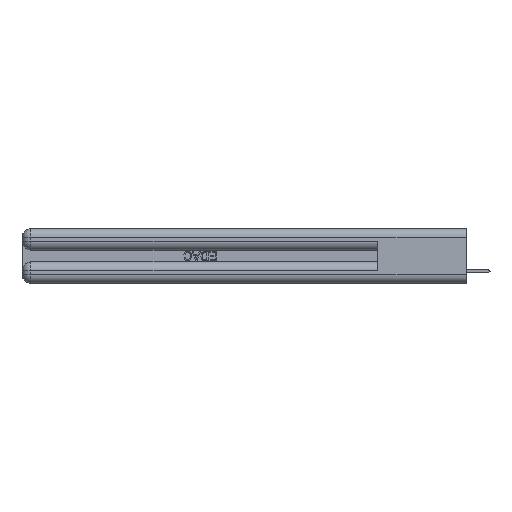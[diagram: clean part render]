
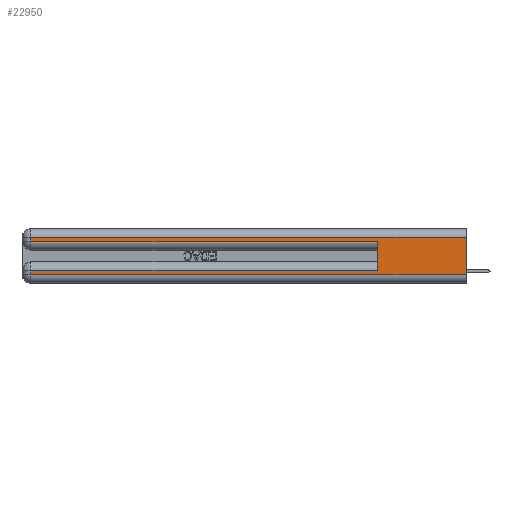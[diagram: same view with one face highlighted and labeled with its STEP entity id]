
A CAD part, left-side view. The second image highlights one B-rep face of the part: STEP entity #22950.
In plain terms, the highlighted planar face has unit normal (-1, 0, 0).
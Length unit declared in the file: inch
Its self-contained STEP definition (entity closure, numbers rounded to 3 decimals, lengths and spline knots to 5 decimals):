
#472 = VERTEX_POINT ( 'NONE', #10232 ) ;
#1618 = EDGE_CURVE ( 'NONE', #12136, #7653, #22465, .T. ) ;
#2491 = EDGE_CURVE ( 'NONE', #32890, #4800, #25394, .T. ) ;
#2884 = LINE ( 'NONE', #32475, #22380 ) ;
#3123 = ORIENTED_EDGE ( 'NONE', *, *, #44836, .T. ) ;
#4800 = VERTEX_POINT ( 'NONE', #15359 ) ;
#6401 = VECTOR ( 'NONE', #38782, 39.37008 ) ;
#7573 = CARTESIAN_POINT ( 'NONE',  ( 0., 0., 0.31 ) ) ;
#7620 = EDGE_CURVE ( 'NONE', #43813, #11728, #45019, .T. ) ;
#7653 = VERTEX_POINT ( 'NONE', #28448 ) ;
#7693 = VECTOR ( 'NONE', #48234, 39.37008 ) ;
#7734 = ORIENTED_EDGE ( 'NONE', *, *, #7620, .F. ) ;
#8067 = EDGE_CURVE ( 'NONE', #43813, #472, #2884, .T. ) ;
#9024 = VECTOR ( 'NONE', #41724, 39.37008 ) ;
#9130 = DIRECTION ( 'NONE',  ( 0., 0., 1. ) ) ;
#10232 = CARTESIAN_POINT ( 'NONE',  ( 0., 2.94, 0.085 ) ) ;
#10291 = CARTESIAN_POINT ( 'NONE',  ( 0., 0., 0.285 ) ) ;
#11388 = ORIENTED_EDGE ( 'NONE', *, *, #48980, .T. ) ;
#11521 = CARTESIAN_POINT ( 'NONE',  ( 0., 2.94, 0.37 ) ) ;
#11728 = VERTEX_POINT ( 'NONE', #25226 ) ;
#11809 = DIRECTION ( 'NONE',  ( 0., 0., -1. ) ) ;
#12136 = VERTEX_POINT ( 'NONE', #29131 ) ;
#12540 = VECTOR ( 'NONE', #37598, 39.37008 ) ;
#12962 = ORIENTED_EDGE ( 'NONE', *, *, #1618, .T. ) ;
#13053 = AXIS2_PLACEMENT_3D ( 'NONE', #23582, #27526, #11809 ) ;
#15359 = CARTESIAN_POINT ( 'NONE',  ( 0., 2.94, 0.31 ) ) ;
#15854 = CARTESIAN_POINT ( 'NONE',  ( 0., 0., 0.31 ) ) ;
#16496 = FACE_OUTER_BOUND ( 'NONE', #35497, .T. ) ;
#20216 = VECTOR ( 'NONE', #34841, 39.37008 ) ;
#22380 = VECTOR ( 'NONE', #36367, 39.37008 ) ;
#22465 = LINE ( 'NONE', #25725, #9024 ) ;
#22947 = LINE ( 'NONE', #10291, #12540 ) ;
#22950 = ADVANCED_FACE ( 'NONE', ( #16496 ), #30790, .F. ) ;
#23055 = VECTOR ( 'NONE', #9130, 39.37008 ) ;
#23582 = CARTESIAN_POINT ( 'NONE',  ( 0., 0., 0.37 ) ) ;
#25226 = CARTESIAN_POINT ( 'NONE',  ( 0., 0.6, 0.285 ) ) ;
#25394 = LINE ( 'NONE', #7573, #26610 ) ;
#25725 = CARTESIAN_POINT ( 'NONE',  ( 0., 0., 0.06 ) ) ;
#26610 = VECTOR ( 'NONE', #38738, 39.37008 ) ;
#27010 = CARTESIAN_POINT ( 'NONE',  ( 0., 2.94, 0.37 ) ) ;
#27526 = DIRECTION ( 'NONE',  ( 1., 0., 0. ) ) ;
#28158 = LINE ( 'NONE', #27010, #20216 ) ;
#28375 = LINE ( 'NONE', #11521, #6401 ) ;
#28448 = CARTESIAN_POINT ( 'NONE',  ( 0., 0., 0.06 ) ) ;
#28781 = ORIENTED_EDGE ( 'NONE', *, *, #2491, .T. ) ;
#29131 = CARTESIAN_POINT ( 'NONE',  ( 0., 2.94, 0.06 ) ) ;
#29298 = EDGE_CURVE ( 'NONE', #48943, #11728, #22947, .T. ) ;
#30790 = PLANE ( 'NONE',  #13053 ) ;
#32175 = ORIENTED_EDGE ( 'NONE', *, *, #29298, .T. ) ;
#32475 = CARTESIAN_POINT ( 'NONE',  ( 0., 0., 0.085 ) ) ;
#32890 = VERTEX_POINT ( 'NONE', #15854 ) ;
#34841 = DIRECTION ( 'NONE',  ( 0., 0., -1. ) ) ;
#35038 = CARTESIAN_POINT ( 'NONE',  ( 0., 2.94, 0.285 ) ) ;
#35497 = EDGE_LOOP ( 'NONE', ( #49540, #28781, #11388, #32175, #7734, #41352, #3123, #12962 ) ) ;
#36367 = DIRECTION ( 'NONE',  ( 0., 1., 0. ) ) ;
#36982 = CARTESIAN_POINT ( 'NONE',  ( 0., 0.6, 0.085 ) ) ;
#37598 = DIRECTION ( 'NONE',  ( 0., -1., 0. ) ) ;
#38738 = DIRECTION ( 'NONE',  ( 0., 1., 0. ) ) ;
#38779 = LINE ( 'NONE', #48405, #7693 ) ;
#38782 = DIRECTION ( 'NONE',  ( 0., 0., -1. ) ) ;
#39975 = CARTESIAN_POINT ( 'NONE',  ( 0., 0.6, 0.145 ) ) ;
#41352 = ORIENTED_EDGE ( 'NONE', *, *, #8067, .T. ) ;
#41724 = DIRECTION ( 'NONE',  ( 0., -1., 0. ) ) ;
#43813 = VERTEX_POINT ( 'NONE', #36982 ) ;
#44836 = EDGE_CURVE ( 'NONE', #472, #12136, #28158, .T. ) ;
#45019 = LINE ( 'NONE', #39975, #23055 ) ;
#47929 = EDGE_CURVE ( 'NONE', #32890, #7653, #38779, .T. ) ;
#48234 = DIRECTION ( 'NONE',  ( 0., 0., -1. ) ) ;
#48405 = CARTESIAN_POINT ( 'NONE',  ( 0., 0., 0.37 ) ) ;
#48943 = VERTEX_POINT ( 'NONE', #35038 ) ;
#48980 = EDGE_CURVE ( 'NONE', #4800, #48943, #28375, .T. ) ;
#49540 = ORIENTED_EDGE ( 'NONE', *, *, #47929, .F. ) ;
